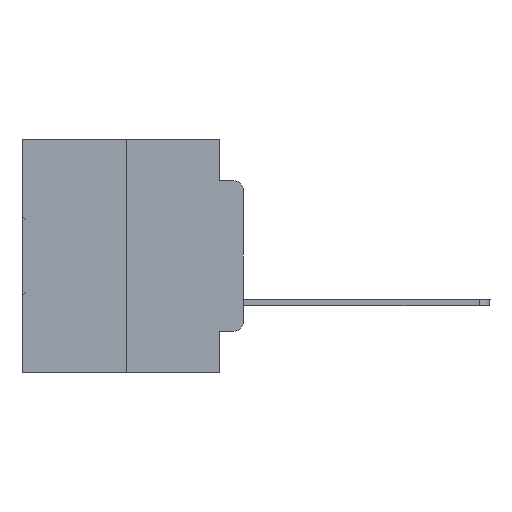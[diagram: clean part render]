
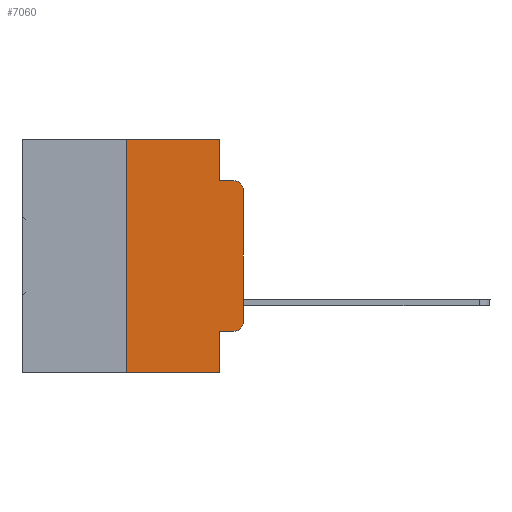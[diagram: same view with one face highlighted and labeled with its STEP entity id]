
A CAD part, left-side view. The second image highlights one B-rep face of the part: STEP entity #7060.
In plain terms, the highlighted planar face has unit normal (-1, 0, 0).
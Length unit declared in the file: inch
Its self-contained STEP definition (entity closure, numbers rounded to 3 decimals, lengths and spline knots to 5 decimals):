
#122 = VECTOR ( 'NONE', #29559, 39.37008 ) ;
#131 = DIRECTION ( 'NONE',  ( 0., 0., 1. ) ) ;
#501 = VERTEX_POINT ( 'NONE', #10359 ) ;
#814 = DIRECTION ( 'NONE',  ( 0., 0., -1. ) ) ;
#941 = LINE ( 'NONE', #23162, #23710 ) ;
#1107 = VECTOR ( 'NONE', #32706, 39.37008 ) ;
#1706 = DIRECTION ( 'NONE',  ( 0., -1., 0. ) ) ;
#2420 = ORIENTED_EDGE ( 'NONE', *, *, #20713, .T. ) ;
#2980 = CIRCLE ( 'NONE', #25232, 0.02 ) ;
#3031 = ORIENTED_EDGE ( 'NONE', *, *, #29235, .F. ) ;
#3377 = DIRECTION ( 'NONE',  ( -1., 0., 0. ) ) ;
#4618 = DIRECTION ( 'NONE',  ( 0., -1., 0. ) ) ;
#5135 = EDGE_LOOP ( 'NONE', ( #6667, #2420, #27931, #13841, #28645, #9988, #15246, #3031, #20440, #20979 ) ) ;
#6134 = CARTESIAN_POINT ( 'NONE',  ( 0., 0.25, 0. ) ) ;
#6519 = CARTESIAN_POINT ( 'NONE',  ( 0., 0.02, -0.0885 ) ) ;
#6667 = ORIENTED_EDGE ( 'NONE', *, *, #30609, .T. ) ;
#7060 = ADVANCED_FACE ( 'NONE', ( #18869 ), #28716, .F. ) ;
#7622 = CIRCLE ( 'NONE', #27985, 0.02 ) ;
#7781 = CARTESIAN_POINT ( 'NONE',  ( 0., 0.051, 0. ) ) ;
#7913 = LINE ( 'NONE', #9631, #1107 ) ;
#8312 = CARTESIAN_POINT ( 'NONE',  ( 0., 0.473, 0. ) ) ;
#8448 = CARTESIAN_POINT ( 'NONE',  ( 0., 0.051, -0.0885 ) ) ;
#8814 = EDGE_CURVE ( 'NONE', #501, #24996, #25852, .T. ) ;
#9631 = CARTESIAN_POINT ( 'NONE',  ( 0., 0.051, 0. ) ) ;
#9847 = EDGE_CURVE ( 'NONE', #27709, #20800, #7913, .T. ) ;
#9988 = ORIENTED_EDGE ( 'NONE', *, *, #22426, .F. ) ;
#10033 = DIRECTION ( 'NONE',  ( 0., 0., -1. ) ) ;
#10126 = DIRECTION ( 'NONE',  ( 0., 0., -1. ) ) ;
#10173 = CARTESIAN_POINT ( 'NONE',  ( 0., 0.051, -0.4115 ) ) ;
#10193 = CARTESIAN_POINT ( 'NONE',  ( 0., 0.051, -0.5 ) ) ;
#10359 = CARTESIAN_POINT ( 'NONE',  ( 0., 0.25, -0.5 ) ) ;
#10483 = CARTESIAN_POINT ( 'NONE',  ( 0., 0.02, -0.4115 ) ) ;
#10721 = VERTEX_POINT ( 'NONE', #19036 ) ;
#10746 = DIRECTION ( 'NONE',  ( 1., 0., 0. ) ) ;
#11444 = VERTEX_POINT ( 'NONE', #12622 ) ;
#12622 = CARTESIAN_POINT ( 'NONE',  ( 0., 0.051, -0.4115 ) ) ;
#12814 = LINE ( 'NONE', #7781, #19629 ) ;
#12924 = CARTESIAN_POINT ( 'NONE',  ( 0., 0.02, -0.3915 ) ) ;
#13293 = CARTESIAN_POINT ( 'NONE',  ( 0., 0., 0. ) ) ;
#13516 = VECTOR ( 'NONE', #131, 39.37008 ) ;
#13530 = CARTESIAN_POINT ( 'NONE',  ( 0., 0., -0.1085 ) ) ;
#13841 = ORIENTED_EDGE ( 'NONE', *, *, #9847, .F. ) ;
#14339 = AXIS2_PLACEMENT_3D ( 'NONE', #8312, #10746, #31074 ) ;
#15246 = ORIENTED_EDGE ( 'NONE', *, *, #8814, .T. ) ;
#15515 = DIRECTION ( 'NONE',  ( 0., -1., 0. ) ) ;
#15726 = VECTOR ( 'NONE', #28031, 39.37008 ) ;
#18034 = EDGE_CURVE ( 'NONE', #22612, #27709, #21461, .T. ) ;
#18285 = LINE ( 'NONE', #13293, #13516 ) ;
#18465 = EDGE_CURVE ( 'NONE', #25141, #10721, #7622, .T. ) ;
#18869 = FACE_OUTER_BOUND ( 'NONE', #5135, .T. ) ;
#19036 = CARTESIAN_POINT ( 'NONE',  ( 0., 0., -0.3915 ) ) ;
#19629 = VECTOR ( 'NONE', #10033, 39.37008 ) ;
#20009 = CARTESIAN_POINT ( 'NONE',  ( 0., 0.473, 0. ) ) ;
#20440 = ORIENTED_EDGE ( 'NONE', *, *, #26911, .T. ) ;
#20713 = EDGE_CURVE ( 'NONE', #27003, #28524, #2980, .T. ) ;
#20800 = VERTEX_POINT ( 'NONE', #8448 ) ;
#20842 = CARTESIAN_POINT ( 'NONE',  ( 0., 0.051, 0. ) ) ;
#20979 = ORIENTED_EDGE ( 'NONE', *, *, #18465, .T. ) ;
#21404 = EDGE_CURVE ( 'NONE', #20800, #28524, #941, .T. ) ;
#21461 = LINE ( 'NONE', #20009, #28223 ) ;
#22110 = LINE ( 'NONE', #6134, #122 ) ;
#22426 = EDGE_CURVE ( 'NONE', #501, #22612, #22110, .T. ) ;
#22612 = VERTEX_POINT ( 'NONE', #27632 ) ;
#23162 = CARTESIAN_POINT ( 'NONE',  ( 0., 0.051, -0.0885 ) ) ;
#23465 = VECTOR ( 'NONE', #1706, 39.37008 ) ;
#23710 = VECTOR ( 'NONE', #15515, 39.37008 ) ;
#24130 = CARTESIAN_POINT ( 'NONE',  ( 0., 0.02, -0.1085 ) ) ;
#24996 = VERTEX_POINT ( 'NONE', #10193 ) ;
#25141 = VERTEX_POINT ( 'NONE', #10483 ) ;
#25232 = AXIS2_PLACEMENT_3D ( 'NONE', #24130, #3377, #814 ) ;
#25852 = LINE ( 'NONE', #30054, #23465 ) ;
#26035 = LINE ( 'NONE', #10173, #15726 ) ;
#26911 = EDGE_CURVE ( 'NONE', #11444, #25141, #26035, .T. ) ;
#27003 = VERTEX_POINT ( 'NONE', #13530 ) ;
#27632 = CARTESIAN_POINT ( 'NONE',  ( 0., 0.25, 0. ) ) ;
#27709 = VERTEX_POINT ( 'NONE', #20842 ) ;
#27931 = ORIENTED_EDGE ( 'NONE', *, *, #21404, .F. ) ;
#27985 = AXIS2_PLACEMENT_3D ( 'NONE', #12924, #30876, #10126 ) ;
#28031 = DIRECTION ( 'NONE',  ( 0., -1., 0. ) ) ;
#28223 = VECTOR ( 'NONE', #4618, 39.37008 ) ;
#28524 = VERTEX_POINT ( 'NONE', #6519 ) ;
#28645 = ORIENTED_EDGE ( 'NONE', *, *, #18034, .F. ) ;
#28716 = PLANE ( 'NONE',  #14339 ) ;
#29235 = EDGE_CURVE ( 'NONE', #11444, #24996, #12814, .T. ) ;
#29559 = DIRECTION ( 'NONE',  ( 0., 0., 1. ) ) ;
#30054 = CARTESIAN_POINT ( 'NONE',  ( 0., 0.473, -0.5 ) ) ;
#30609 = EDGE_CURVE ( 'NONE', #10721, #27003, #18285, .T. ) ;
#30876 = DIRECTION ( 'NONE',  ( -1., 0., 0. ) ) ;
#31074 = DIRECTION ( 'NONE',  ( 0., 0., -1. ) ) ;
#32706 = DIRECTION ( 'NONE',  ( 0., 0., -1. ) ) ;
